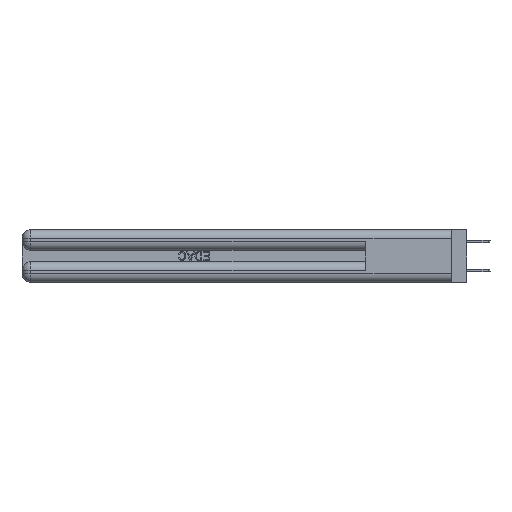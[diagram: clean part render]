
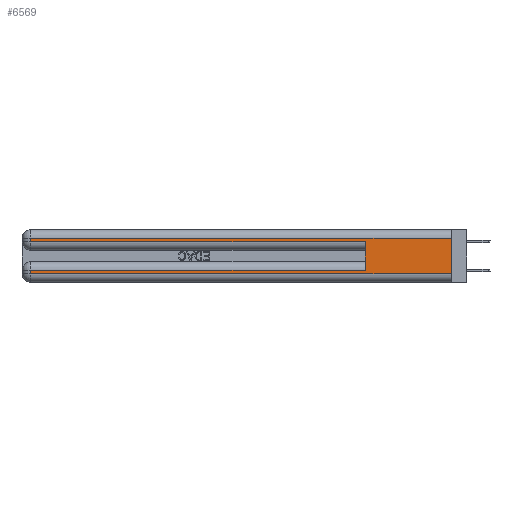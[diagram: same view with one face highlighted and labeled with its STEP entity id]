
A CAD part, left-side view. The second image highlights one B-rep face of the part: STEP entity #6569.
In plain terms, the highlighted planar face has unit normal (-1, 0, 0).
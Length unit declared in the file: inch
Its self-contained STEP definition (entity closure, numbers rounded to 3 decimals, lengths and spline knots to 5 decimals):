
#88 = LINE ( 'NONE', #45918, #50361 ) ;
#307 = LINE ( 'NONE', #16575, #9493 ) ;
#722 = LINE ( 'NONE', #2025, #38707 ) ;
#1232 = VERTEX_POINT ( 'NONE', #37638 ) ;
#1846 = CARTESIAN_POINT ( 'NONE',  ( 0., 0.6, 0.285 ) ) ;
#1885 = CARTESIAN_POINT ( 'NONE',  ( 0., 0., 0.06 ) ) ;
#2025 = CARTESIAN_POINT ( 'NONE',  ( 0., 0., 0.285 ) ) ;
#6338 = VERTEX_POINT ( 'NONE', #29259 ) ;
#6569 = ADVANCED_FACE ( 'NONE', ( #25313 ), #23277, .F. ) ;
#7816 = VERTEX_POINT ( 'NONE', #15289 ) ;
#7817 = DIRECTION ( 'NONE',  ( 1., 0., 0. ) ) ;
#8024 = ORIENTED_EDGE ( 'NONE', *, *, #41221, .T. ) ;
#9493 = VECTOR ( 'NONE', #20170, 39.37008 ) ;
#11598 = ORIENTED_EDGE ( 'NONE', *, *, #19749, .T. ) ;
#11963 = DIRECTION ( 'NONE',  ( 0., 1., 0. ) ) ;
#12408 = EDGE_CURVE ( 'NONE', #1232, #15218, #88, .T. ) ;
#15218 = VERTEX_POINT ( 'NONE', #19331 ) ;
#15289 = CARTESIAN_POINT ( 'NONE',  ( 0., 0.6, 0.085 ) ) ;
#15895 = LINE ( 'NONE', #1885, #42804 ) ;
#15914 = DIRECTION ( 'NONE',  ( 0., 0., -1. ) ) ;
#16270 = CARTESIAN_POINT ( 'NONE',  ( 0., 2.94, 0.285 ) ) ;
#16424 = ORIENTED_EDGE ( 'NONE', *, *, #38035, .F. ) ;
#16575 = CARTESIAN_POINT ( 'NONE',  ( 0., 0.6, 0.145 ) ) ;
#16956 = ORIENTED_EDGE ( 'NONE', *, *, #19677, .T. ) ;
#17983 = VECTOR ( 'NONE', #15914, 39.37008 ) ;
#18186 = AXIS2_PLACEMENT_3D ( 'NONE', #23772, #7817, #43243 ) ;
#18459 = CARTESIAN_POINT ( 'NONE',  ( 0., 0., 0.37 ) ) ;
#18841 = DIRECTION ( 'NONE',  ( 0., 1., 0. ) ) ;
#18847 = CARTESIAN_POINT ( 'NONE',  ( 0., 0., 0.31 ) ) ;
#19041 = VERTEX_POINT ( 'NONE', #42326 ) ;
#19331 = CARTESIAN_POINT ( 'NONE',  ( 0., 2.94, 0.06 ) ) ;
#19677 = EDGE_CURVE ( 'NONE', #6338, #19041, #20364, .T. ) ;
#19749 = EDGE_CURVE ( 'NONE', #37673, #23256, #722, .T. ) ;
#20170 = DIRECTION ( 'NONE',  ( 0., 0., 1. ) ) ;
#20364 = LINE ( 'NONE', #18847, #39907 ) ;
#22386 = LINE ( 'NONE', #41912, #46245 ) ;
#23256 = VERTEX_POINT ( 'NONE', #1846 ) ;
#23277 = PLANE ( 'NONE',  #18186 ) ;
#23772 = CARTESIAN_POINT ( 'NONE',  ( 0., 0., 0.37 ) ) ;
#25054 = VERTEX_POINT ( 'NONE', #44660 ) ;
#25313 = FACE_OUTER_BOUND ( 'NONE', #31113, .T. ) ;
#26723 = DIRECTION ( 'NONE',  ( 0., 0., -1. ) ) ;
#29033 = ORIENTED_EDGE ( 'NONE', *, *, #12408, .T. ) ;
#29259 = CARTESIAN_POINT ( 'NONE',  ( 0., 0., 0.31 ) ) ;
#29810 = ORIENTED_EDGE ( 'NONE', *, *, #34527, .T. ) ;
#31113 = EDGE_LOOP ( 'NONE', ( #16424, #16956, #8024, #11598, #48894, #29810, #29033, #31737 ) ) ;
#31737 = ORIENTED_EDGE ( 'NONE', *, *, #44506, .T. ) ;
#34261 = DIRECTION ( 'NONE',  ( 0., 0., -1. ) ) ;
#34527 = EDGE_CURVE ( 'NONE', #7816, #1232, #22386, .T. ) ;
#35794 = LINE ( 'NONE', #37708, #37021 ) ;
#37021 = VECTOR ( 'NONE', #26723, 39.37008 ) ;
#37638 = CARTESIAN_POINT ( 'NONE',  ( 0., 2.94, 0.085 ) ) ;
#37673 = VERTEX_POINT ( 'NONE', #16270 ) ;
#37708 = CARTESIAN_POINT ( 'NONE',  ( 0., 2.94, 0.37 ) ) ;
#38035 = EDGE_CURVE ( 'NONE', #6338, #25054, #39985, .T. ) ;
#38707 = VECTOR ( 'NONE', #44305, 39.37008 ) ;
#39907 = VECTOR ( 'NONE', #11963, 39.37008 ) ;
#39985 = LINE ( 'NONE', #18459, #17983 ) ;
#41221 = EDGE_CURVE ( 'NONE', #19041, #37673, #35794, .T. ) ;
#41912 = CARTESIAN_POINT ( 'NONE',  ( 0., 0., 0.085 ) ) ;
#42326 = CARTESIAN_POINT ( 'NONE',  ( 0., 2.94, 0.31 ) ) ;
#42804 = VECTOR ( 'NONE', #44865, 39.37008 ) ;
#43243 = DIRECTION ( 'NONE',  ( 0., 0., -1. ) ) ;
#44305 = DIRECTION ( 'NONE',  ( 0., -1., 0. ) ) ;
#44506 = EDGE_CURVE ( 'NONE', #15218, #25054, #15895, .T. ) ;
#44660 = CARTESIAN_POINT ( 'NONE',  ( 0., 0., 0.06 ) ) ;
#44865 = DIRECTION ( 'NONE',  ( 0., -1., 0. ) ) ;
#45918 = CARTESIAN_POINT ( 'NONE',  ( 0., 2.94, 0.37 ) ) ;
#46245 = VECTOR ( 'NONE', #18841, 39.37008 ) ;
#46547 = EDGE_CURVE ( 'NONE', #7816, #23256, #307, .T. ) ;
#48894 = ORIENTED_EDGE ( 'NONE', *, *, #46547, .F. ) ;
#50361 = VECTOR ( 'NONE', #34261, 39.37008 ) ;
